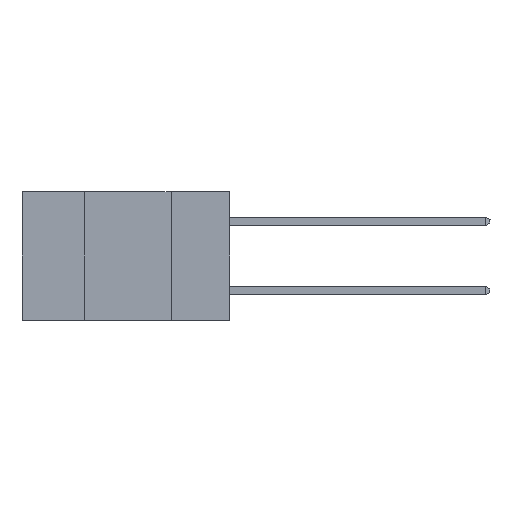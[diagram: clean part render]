
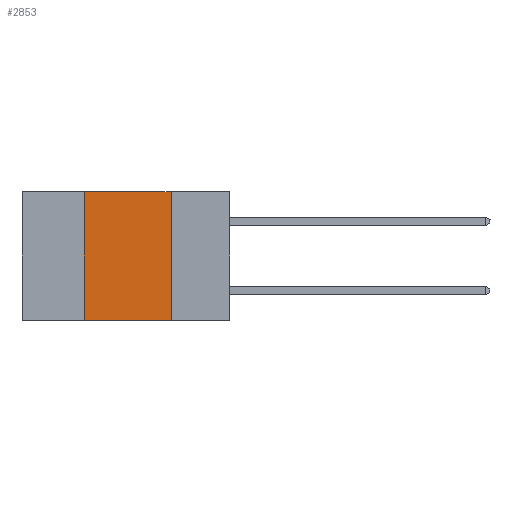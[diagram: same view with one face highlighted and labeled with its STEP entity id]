
A CAD part, left-side view. The second image highlights one B-rep face of the part: STEP entity #2853.
In plain terms, the highlighted planar face has unit normal (-1, 0, 0).
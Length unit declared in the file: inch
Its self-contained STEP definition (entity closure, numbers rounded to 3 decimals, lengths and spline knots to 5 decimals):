
#132 = DIRECTION ( 'NONE',  ( 0., -1., 0. ) ) ;
#179 = VERTEX_POINT ( 'NONE', #9574 ) ;
#477 = CARTESIAN_POINT ( 'NONE',  ( 0., 0.17, 0. ) ) ;
#535 = PLANE ( 'NONE',  #5722 ) ;
#624 = EDGE_LOOP ( 'NONE', ( #2784, #3625, #7351, #8564 ) ) ;
#834 = CARTESIAN_POINT ( 'NONE',  ( 0., 0.17, -0.37 ) ) ;
#1608 = DIRECTION ( 'NONE',  ( 0., 0., -1. ) ) ;
#2401 = EDGE_CURVE ( 'NONE', #3595, #179, #8242, .T. ) ;
#2764 = FACE_OUTER_BOUND ( 'NONE', #624, .T. ) ;
#2784 = ORIENTED_EDGE ( 'NONE', *, *, #9165, .F. ) ;
#2853 = ADVANCED_FACE ( 'NONE', ( #2764 ), #535, .F. ) ;
#3034 = CARTESIAN_POINT ( 'NONE',  ( 0., 0.42, -0.37 ) ) ;
#3492 = VERTEX_POINT ( 'NONE', #5441 ) ;
#3595 = VERTEX_POINT ( 'NONE', #9622 ) ;
#3625 = ORIENTED_EDGE ( 'NONE', *, *, #6772, .F. ) ;
#3822 = CARTESIAN_POINT ( 'NONE',  ( 0., 0.6, -0.37 ) ) ;
#3971 = DIRECTION ( 'NONE',  ( 0., 0., 1. ) ) ;
#4319 = VECTOR ( 'NONE', #132, 39.37008 ) ;
#4593 = LINE ( 'NONE', #5254, #7673 ) ;
#5254 = CARTESIAN_POINT ( 'NONE',  ( 0., 0.6, 0. ) ) ;
#5317 = VECTOR ( 'NONE', #1608, 39.37008 ) ;
#5441 = CARTESIAN_POINT ( 'NONE',  ( 0., 0.42, 0. ) ) ;
#5722 = AXIS2_PLACEMENT_3D ( 'NONE', #9366, #7810, #9311 ) ;
#6124 = DIRECTION ( 'NONE',  ( 0., -1., 0. ) ) ;
#6772 = EDGE_CURVE ( 'NONE', #3492, #7915, #4593, .T. ) ;
#7351 = ORIENTED_EDGE ( 'NONE', *, *, #9067, .F. ) ;
#7567 = LINE ( 'NONE', #834, #5317 ) ;
#7673 = VECTOR ( 'NONE', #6124, 39.37008 ) ;
#7810 = DIRECTION ( 'NONE',  ( 1., 0., 0. ) ) ;
#7915 = VERTEX_POINT ( 'NONE', #477 ) ;
#8242 = LINE ( 'NONE', #3822, #4319 ) ;
#8564 = ORIENTED_EDGE ( 'NONE', *, *, #2401, .T. ) ;
#9067 = EDGE_CURVE ( 'NONE', #3595, #3492, #9201, .T. ) ;
#9092 = VECTOR ( 'NONE', #3971, 39.37008 ) ;
#9165 = EDGE_CURVE ( 'NONE', #7915, #179, #7567, .T. ) ;
#9201 = LINE ( 'NONE', #3034, #9092 ) ;
#9311 = DIRECTION ( 'NONE',  ( 0., 0., -1. ) ) ;
#9366 = CARTESIAN_POINT ( 'NONE',  ( 0., 0.6, 0. ) ) ;
#9574 = CARTESIAN_POINT ( 'NONE',  ( 0., 0.17, -0.37 ) ) ;
#9622 = CARTESIAN_POINT ( 'NONE',  ( 0., 0.42, -0.37 ) ) ;
